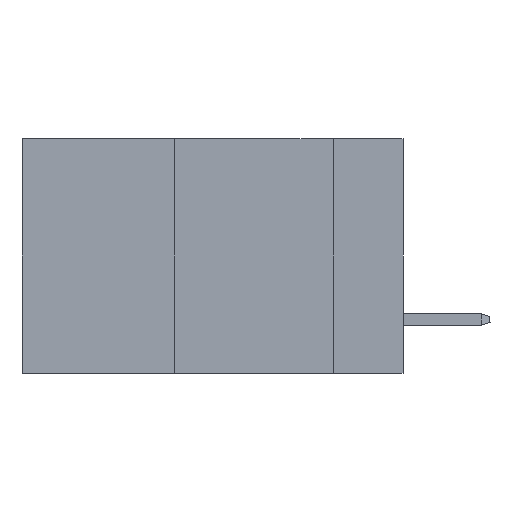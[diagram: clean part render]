
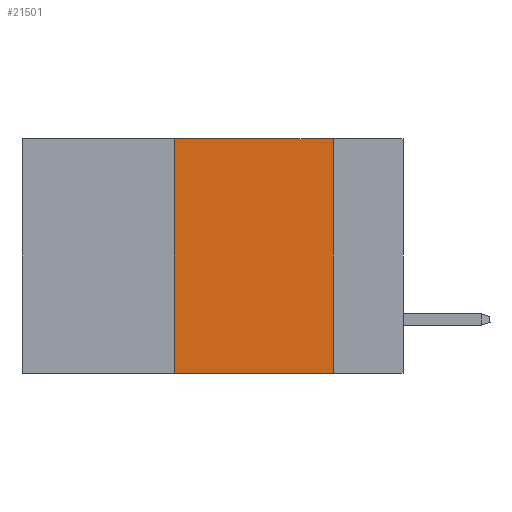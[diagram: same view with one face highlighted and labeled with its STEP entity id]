
A CAD part, left-side view. The second image highlights one B-rep face of the part: STEP entity #21501.
In plain terms, the highlighted planar face has unit normal (-1, 0, 0).
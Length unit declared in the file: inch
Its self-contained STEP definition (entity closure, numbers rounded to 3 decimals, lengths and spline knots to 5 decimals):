
#329 = DIRECTION ( 'NONE',  ( 1., 0., 0. ) ) ;
#542 = PLANE ( 'NONE',  #27973 ) ;
#678 = VECTOR ( 'NONE', #28391, 39.37008 ) ;
#2709 = LINE ( 'NONE', #37589, #43948 ) ;
#4434 = FACE_OUTER_BOUND ( 'NONE', #9276, .T. ) ;
#6041 = EDGE_CURVE ( 'NONE', #6755, #14061, #21317, .T. ) ;
#6755 = VERTEX_POINT ( 'NONE', #42125 ) ;
#7695 = ORIENTED_EDGE ( 'NONE', *, *, #6041, .T. ) ;
#8006 = VECTOR ( 'NONE', #32157, 39.37008 ) ;
#8415 = ORIENTED_EDGE ( 'NONE', *, *, #41220, .F. ) ;
#9276 = EDGE_LOOP ( 'NONE', ( #8415, #15326, #17128, #7695 ) ) ;
#10966 = LINE ( 'NONE', #11418, #678 ) ;
#11418 = CARTESIAN_POINT ( 'NONE',  ( 0., 0.36, 0. ) ) ;
#11765 = CARTESIAN_POINT ( 'NONE',  ( 0., 0.11, -0.37 ) ) ;
#14061 = VERTEX_POINT ( 'NONE', #11765 ) ;
#14887 = EDGE_CURVE ( 'NONE', #6755, #28114, #10966, .T. ) ;
#15194 = CARTESIAN_POINT ( 'NONE',  ( 0., 0.6, 0. ) ) ;
#15250 = EDGE_CURVE ( 'NONE', #28114, #36308, #2709, .T. ) ;
#15326 = ORIENTED_EDGE ( 'NONE', *, *, #15250, .F. ) ;
#17128 = ORIENTED_EDGE ( 'NONE', *, *, #14887, .F. ) ;
#18637 = DIRECTION ( 'NONE',  ( 0., 0., -1. ) ) ;
#19985 = CARTESIAN_POINT ( 'NONE',  ( 0., 0.11, 0. ) ) ;
#21317 = LINE ( 'NONE', #28450, #45122 ) ;
#21501 = ADVANCED_FACE ( 'NONE', ( #4434 ), #542, .F. ) ;
#24779 = DIRECTION ( 'NONE',  ( 0., -1., 0. ) ) ;
#25255 = LINE ( 'NONE', #32849, #8006 ) ;
#26989 = DIRECTION ( 'NONE',  ( 0., -1., 0. ) ) ;
#27973 = AXIS2_PLACEMENT_3D ( 'NONE', #15194, #329, #18637 ) ;
#28114 = VERTEX_POINT ( 'NONE', #38120 ) ;
#28391 = DIRECTION ( 'NONE',  ( 0., 0., 1. ) ) ;
#28450 = CARTESIAN_POINT ( 'NONE',  ( 0., 0.6, -0.37 ) ) ;
#32157 = DIRECTION ( 'NONE',  ( 0., 0., -1. ) ) ;
#32849 = CARTESIAN_POINT ( 'NONE',  ( 0., 0.11, 0. ) ) ;
#36308 = VERTEX_POINT ( 'NONE', #19985 ) ;
#37589 = CARTESIAN_POINT ( 'NONE',  ( 0., 0.6, 0. ) ) ;
#38120 = CARTESIAN_POINT ( 'NONE',  ( 0., 0.36, 0. ) ) ;
#41220 = EDGE_CURVE ( 'NONE', #36308, #14061, #25255, .T. ) ;
#42125 = CARTESIAN_POINT ( 'NONE',  ( 0., 0.36, -0.37 ) ) ;
#43948 = VECTOR ( 'NONE', #26989, 39.37008 ) ;
#45122 = VECTOR ( 'NONE', #24779, 39.37008 ) ;
